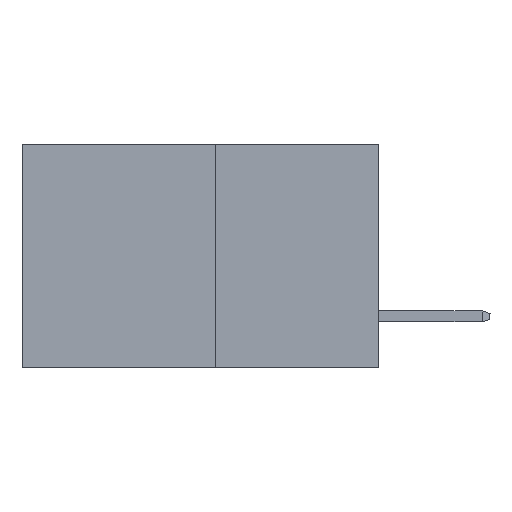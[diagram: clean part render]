
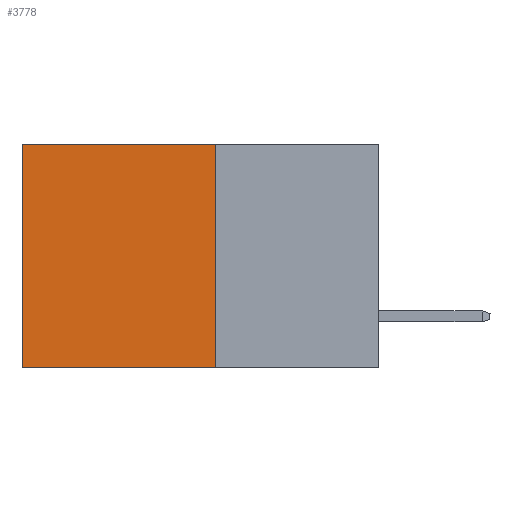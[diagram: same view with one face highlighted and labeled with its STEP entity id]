
A CAD part, left-side view. The second image highlights one B-rep face of the part: STEP entity #3778.
In plain terms, the highlighted planar face has unit normal (-1, 0, 0).
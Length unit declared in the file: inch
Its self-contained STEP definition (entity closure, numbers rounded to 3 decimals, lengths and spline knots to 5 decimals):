
#236 = VERTEX_POINT ( 'NONE', #3978 ) ;
#441 = VECTOR ( 'NONE', #6697, 39.37008 ) ;
#672 = CARTESIAN_POINT ( 'NONE',  ( 0.277, 0.27, -0.37 ) ) ;
#1145 = ORIENTED_EDGE ( 'NONE', *, *, #5964, .T. ) ;
#1616 = DIRECTION ( 'NONE',  ( 0., 1., 0. ) ) ;
#1857 = VERTEX_POINT ( 'NONE', #4892 ) ;
#2179 = VECTOR ( 'NONE', #7799, 39.37008 ) ;
#2327 = CARTESIAN_POINT ( 'NONE',  ( 0.277, 0.59, -0.37 ) ) ;
#2359 = EDGE_CURVE ( 'NONE', #5685, #1857, #5521, .T. ) ;
#2636 = VERTEX_POINT ( 'NONE', #5853 ) ;
#2926 = VECTOR ( 'NONE', #11001, 39.37008 ) ;
#3096 = ORIENTED_EDGE ( 'NONE', *, *, #7581, .T. ) ;
#3204 = AXIS2_PLACEMENT_3D ( 'NONE', #10976, #5789, #5776 ) ;
#3352 = VECTOR ( 'NONE', #1616, 39.37008 ) ;
#3448 = CARTESIAN_POINT ( 'NONE',  ( 0.277, 0.27, 0. ) ) ;
#3665 = LINE ( 'NONE', #3448, #3352 ) ;
#3778 = ADVANCED_FACE ( 'NONE', ( #10636 ), #10996, .F. ) ;
#3978 = CARTESIAN_POINT ( 'NONE',  ( 0.277, 0.27, 0. ) ) ;
#4288 = EDGE_LOOP ( 'NONE', ( #3096, #9459, #9674, #1145 ) ) ;
#4892 = CARTESIAN_POINT ( 'NONE',  ( 0.277, 0.59, -0.37 ) ) ;
#5521 = LINE ( 'NONE', #5647, #2926 ) ;
#5647 = CARTESIAN_POINT ( 'NONE',  ( 0.277, 0.27, -0.37 ) ) ;
#5685 = VERTEX_POINT ( 'NONE', #5689 ) ;
#5689 = CARTESIAN_POINT ( 'NONE',  ( 0.277, 0.27, -0.37 ) ) ;
#5776 = DIRECTION ( 'NONE',  ( 0., 0., -1. ) ) ;
#5789 = DIRECTION ( 'NONE',  ( 1., 0., 0. ) ) ;
#5853 = CARTESIAN_POINT ( 'NONE',  ( 0.277, 0.59, 0. ) ) ;
#5964 = EDGE_CURVE ( 'NONE', #236, #2636, #3665, .T. ) ;
#6697 = DIRECTION ( 'NONE',  ( 0., 0., -1. ) ) ;
#7147 = EDGE_CURVE ( 'NONE', #236, #5685, #8705, .T. ) ;
#7577 = LINE ( 'NONE', #2327, #441 ) ;
#7581 = EDGE_CURVE ( 'NONE', #2636, #1857, #7577, .T. ) ;
#7799 = DIRECTION ( 'NONE',  ( 0., 0., -1. ) ) ;
#8705 = LINE ( 'NONE', #672, #2179 ) ;
#9459 = ORIENTED_EDGE ( 'NONE', *, *, #2359, .F. ) ;
#9674 = ORIENTED_EDGE ( 'NONE', *, *, #7147, .F. ) ;
#10636 = FACE_OUTER_BOUND ( 'NONE', #4288, .T. ) ;
#10976 = CARTESIAN_POINT ( 'NONE',  ( 0.277, 0.27, -0.37 ) ) ;
#10996 = PLANE ( 'NONE',  #3204 ) ;
#11001 = DIRECTION ( 'NONE',  ( 0., 1., 0. ) ) ;
